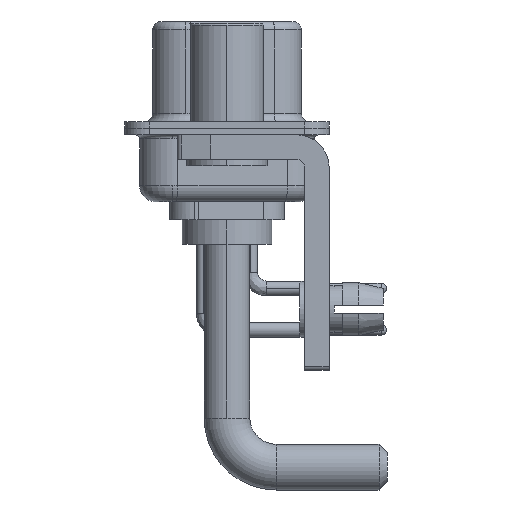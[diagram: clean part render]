
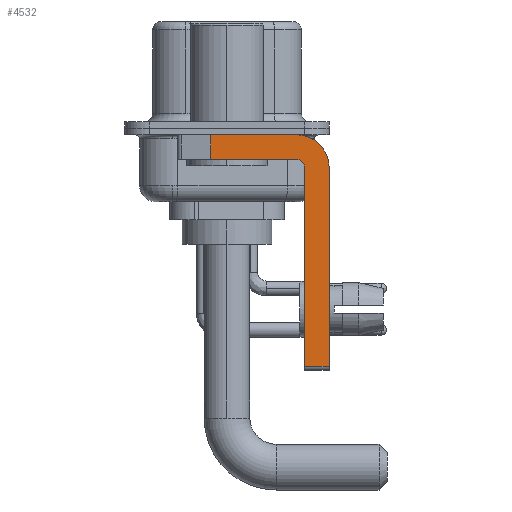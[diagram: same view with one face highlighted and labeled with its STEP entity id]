
A CAD part, left-side view. The second image highlights one B-rep face of the part: STEP entity #4532.
In plain terms, the highlighted planar face has unit normal (-1, 0, 0).
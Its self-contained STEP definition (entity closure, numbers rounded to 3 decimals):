
#198 = VERTEX_POINT ( 'NONE', #13308 ) ;
#761 = DIRECTION ( 'NONE',  ( 0., 0., -1. ) ) ;
#4281 = CIRCLE ( 'NONE', #16027, 2. ) ;
#4292 = ORIENTED_EDGE ( 'NONE', *, *, #19043, .T. ) ;
#4532 = ADVANCED_FACE ( 'NONE', ( #9972 ), #7855, .F. ) ;
#4971 = DIRECTION ( 'NONE',  ( 0., -1., 0. ) ) ;
#5444 = CARTESIAN_POINT ( 'NONE',  ( -2.9, 0.978, -1.9 ) ) ;
#5802 = ORIENTED_EDGE ( 'NONE', *, *, #20737, .F. ) ;
#5938 = DIRECTION ( 'NONE',  ( 0., 0., 1. ) ) ;
#6007 = CARTESIAN_POINT ( 'NONE',  ( -2.9, -4.25, -2.4 ) ) ;
#6061 = CARTESIAN_POINT ( 'NONE',  ( -2.9, -6.25, -2.4 ) ) ;
#6995 = VECTOR ( 'NONE', #17180, 1000. ) ;
#7153 = CARTESIAN_POINT ( 'NONE',  ( -2.9, -4.25, -0.4 ) ) ;
#7399 = EDGE_CURVE ( 'NONE', #18128, #11374, #20004, .T. ) ;
#7855 = PLANE ( 'NONE',  #10334 ) ;
#8092 = CARTESIAN_POINT ( 'NONE',  ( -2.9, 0.978, -0.4 ) ) ;
#8539 = LINE ( 'NONE', #19460, #6995 ) ;
#9972 = FACE_OUTER_BOUND ( 'NONE', #20245, .T. ) ;
#10320 = CARTESIAN_POINT ( 'NONE',  ( -2.9, 0.978, -1.9 ) ) ;
#10334 = AXIS2_PLACEMENT_3D ( 'NONE', #6007, #14631, #16486 ) ;
#10402 = ORIENTED_EDGE ( 'NONE', *, *, #27740, .F. ) ;
#10944 = CARTESIAN_POINT ( 'NONE',  ( -2.9, -4.25, -1.9 ) ) ;
#11199 = ORIENTED_EDGE ( 'NONE', *, *, #7399, .F. ) ;
#11338 = CARTESIAN_POINT ( 'NONE',  ( -2.9, 3., -0.4 ) ) ;
#11374 = VERTEX_POINT ( 'NONE', #25357 ) ;
#12005 = VERTEX_POINT ( 'NONE', #23329 ) ;
#12842 = LINE ( 'NONE', #6061, #26957 ) ;
#13069 = CARTESIAN_POINT ( 'NONE',  ( -2.9, -4.25, -2.4 ) ) ;
#13308 = CARTESIAN_POINT ( 'NONE',  ( -2.9, -6.25, -2.4 ) ) ;
#13348 = DIRECTION ( 'NONE',  ( 0., 1., 0. ) ) ;
#13742 = ORIENTED_EDGE ( 'NONE', *, *, #15327, .F. ) ;
#14400 = VECTOR ( 'NONE', #13348, 1000. ) ;
#14631 = DIRECTION ( 'NONE',  ( 1., 0., 0. ) ) ;
#14696 = LINE ( 'NONE', #21646, #18267 ) ;
#15013 = AXIS2_PLACEMENT_3D ( 'NONE', #20751, #16493, #18900 ) ;
#15299 = EDGE_CURVE ( 'NONE', #12005, #21592, #8539, .T. ) ;
#15327 = EDGE_CURVE ( 'NONE', #27295, #198, #4281, .T. ) ;
#15467 = VERTEX_POINT ( 'NONE', #8092 ) ;
#15673 = ORIENTED_EDGE ( 'NONE', *, *, #24908, .F. ) ;
#16027 = AXIS2_PLACEMENT_3D ( 'NONE', #13069, #21713, #26527 ) ;
#16102 = EDGE_CURVE ( 'NONE', #12005, #18128, #14696, .T. ) ;
#16215 = LINE ( 'NONE', #5444, #27898 ) ;
#16486 = DIRECTION ( 'NONE',  ( 0., 0., -1. ) ) ;
#16493 = DIRECTION ( 'NONE',  ( -1., 0., 0. ) ) ;
#16551 = CARTESIAN_POINT ( 'NONE',  ( -2.9, -4.75, -2.4 ) ) ;
#16680 = DIRECTION ( 'NONE',  ( 0., 0., -1. ) ) ;
#17180 = DIRECTION ( 'NONE',  ( 0., -1., 0. ) ) ;
#18128 = VERTEX_POINT ( 'NONE', #16551 ) ;
#18267 = VECTOR ( 'NONE', #5938, 1000. ) ;
#18769 = ORIENTED_EDGE ( 'NONE', *, *, #16102, .F. ) ;
#18900 = DIRECTION ( 'NONE',  ( 0., 0., 1. ) ) ;
#19043 = EDGE_CURVE ( 'NONE', #15467, #19686, #16215, .T. ) ;
#19460 = CARTESIAN_POINT ( 'NONE',  ( -2.9, -4.25, -14.55 ) ) ;
#19686 = VERTEX_POINT ( 'NONE', #10320 ) ;
#20004 = CIRCLE ( 'NONE', #15013, 0.5 ) ;
#20062 = CARTESIAN_POINT ( 'NONE',  ( -2.9, -6.25, -14.55 ) ) ;
#20245 = EDGE_LOOP ( 'NONE', ( #10402, #4292, #5802, #11199, #18769, #25485, #15673, #13742 ) ) ;
#20737 = EDGE_CURVE ( 'NONE', #11374, #19686, #25988, .T. ) ;
#20751 = CARTESIAN_POINT ( 'NONE',  ( -2.9, -4.25, -2.4 ) ) ;
#21592 = VERTEX_POINT ( 'NONE', #20062 ) ;
#21646 = CARTESIAN_POINT ( 'NONE',  ( -2.9, -4.75, -14.8 ) ) ;
#21713 = DIRECTION ( 'NONE',  ( 1., 0., 0. ) ) ;
#23329 = CARTESIAN_POINT ( 'NONE',  ( -2.9, -4.75, -14.55 ) ) ;
#24421 = LINE ( 'NONE', #11338, #26610 ) ;
#24908 = EDGE_CURVE ( 'NONE', #198, #21592, #12842, .T. ) ;
#25357 = CARTESIAN_POINT ( 'NONE',  ( -2.9, -4.25, -1.9 ) ) ;
#25485 = ORIENTED_EDGE ( 'NONE', *, *, #15299, .T. ) ;
#25988 = LINE ( 'NONE', #10944, #14400 ) ;
#26527 = DIRECTION ( 'NONE',  ( 0., 0., -1. ) ) ;
#26610 = VECTOR ( 'NONE', #4971, 1000. ) ;
#26957 = VECTOR ( 'NONE', #16680, 1000. ) ;
#27295 = VERTEX_POINT ( 'NONE', #7153 ) ;
#27740 = EDGE_CURVE ( 'NONE', #15467, #27295, #24421, .T. ) ;
#27898 = VECTOR ( 'NONE', #761, 1000. ) ;
